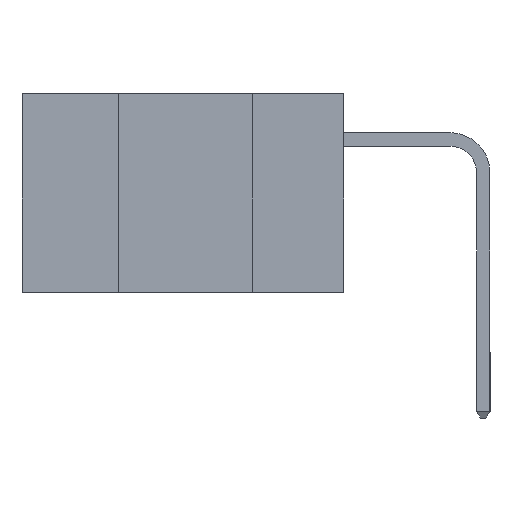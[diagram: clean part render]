
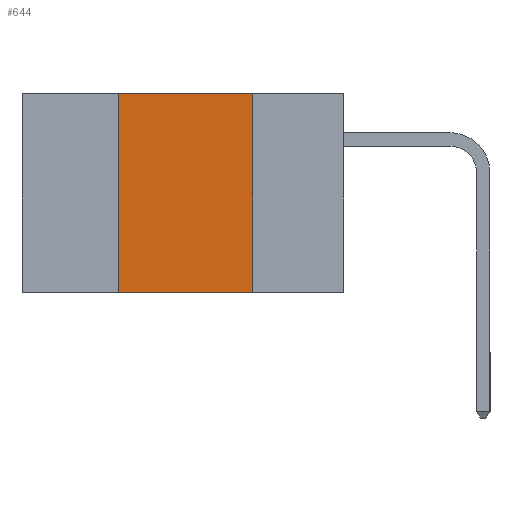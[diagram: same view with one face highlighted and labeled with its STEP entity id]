
A CAD part, left-side view. The second image highlights one B-rep face of the part: STEP entity #644.
In plain terms, the highlighted planar face has unit normal (-1, 0, 0).
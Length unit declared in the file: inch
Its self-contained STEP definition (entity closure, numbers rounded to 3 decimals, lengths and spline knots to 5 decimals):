
#197 = VECTOR ( 'NONE', #1038, 39.37008 ) ;
#527 = VECTOR ( 'NONE', #17277, 39.37008 ) ;
#644 = ADVANCED_FACE ( 'NONE', ( #2884 ), #5362, .F. ) ;
#1003 = VERTEX_POINT ( 'NONE', #16931 ) ;
#1038 = DIRECTION ( 'NONE',  ( 0., -1., 0. ) ) ;
#1466 = DIRECTION ( 'NONE',  ( 1., 0., 0. ) ) ;
#1752 = EDGE_CURVE ( 'NONE', #1003, #6463, #14148, .T. ) ;
#2520 = CARTESIAN_POINT ( 'NONE',  ( 0., 0.17, -0.37 ) ) ;
#2716 = DIRECTION ( 'NONE',  ( 0., 0., 1. ) ) ;
#2884 = FACE_OUTER_BOUND ( 'NONE', #16856, .T. ) ;
#3946 = CARTESIAN_POINT ( 'NONE',  ( 0., 0.6, 0. ) ) ;
#4441 = CARTESIAN_POINT ( 'NONE',  ( 0., 0.17, 0. ) ) ;
#5362 = PLANE ( 'NONE',  #16424 ) ;
#5451 = CARTESIAN_POINT ( 'NONE',  ( 0., 0.42, -0.37 ) ) ;
#5800 = VERTEX_POINT ( 'NONE', #4441 ) ;
#6093 = CARTESIAN_POINT ( 'NONE',  ( 0., 0.42, 0. ) ) ;
#6109 = DIRECTION ( 'NONE',  ( 0., -1., 0. ) ) ;
#6463 = VERTEX_POINT ( 'NONE', #11190 ) ;
#8313 = LINE ( 'NONE', #5451, #16617 ) ;
#9114 = LINE ( 'NONE', #14486, #197 ) ;
#10454 = CARTESIAN_POINT ( 'NONE',  ( 0., 0.6, -0.37 ) ) ;
#11190 = CARTESIAN_POINT ( 'NONE',  ( 0., 0.17, -0.37 ) ) ;
#12349 = VERTEX_POINT ( 'NONE', #6093 ) ;
#12411 = ORIENTED_EDGE ( 'NONE', *, *, #1752, .T. ) ;
#13295 = ORIENTED_EDGE ( 'NONE', *, *, #17396, .F. ) ;
#13805 = ORIENTED_EDGE ( 'NONE', *, *, #15212, .F. ) ;
#14148 = LINE ( 'NONE', #10454, #16162 ) ;
#14486 = CARTESIAN_POINT ( 'NONE',  ( 0., 0.6, 0. ) ) ;
#14900 = DIRECTION ( 'NONE',  ( 0., 0., -1. ) ) ;
#15212 = EDGE_CURVE ( 'NONE', #12349, #5800, #9114, .T. ) ;
#15699 = LINE ( 'NONE', #2520, #527 ) ;
#16162 = VECTOR ( 'NONE', #6109, 39.37008 ) ;
#16424 = AXIS2_PLACEMENT_3D ( 'NONE', #3946, #1466, #14900 ) ;
#16617 = VECTOR ( 'NONE', #2716, 39.37008 ) ;
#16856 = EDGE_LOOP ( 'NONE', ( #13295, #13805, #17389, #12411 ) ) ;
#16931 = CARTESIAN_POINT ( 'NONE',  ( 0., 0.42, -0.37 ) ) ;
#17168 = EDGE_CURVE ( 'NONE', #1003, #12349, #8313, .T. ) ;
#17277 = DIRECTION ( 'NONE',  ( 0., 0., -1. ) ) ;
#17389 = ORIENTED_EDGE ( 'NONE', *, *, #17168, .F. ) ;
#17396 = EDGE_CURVE ( 'NONE', #5800, #6463, #15699, .T. ) ;
